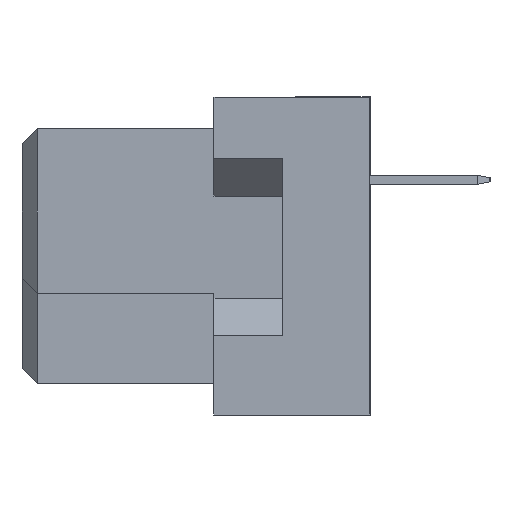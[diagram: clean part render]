
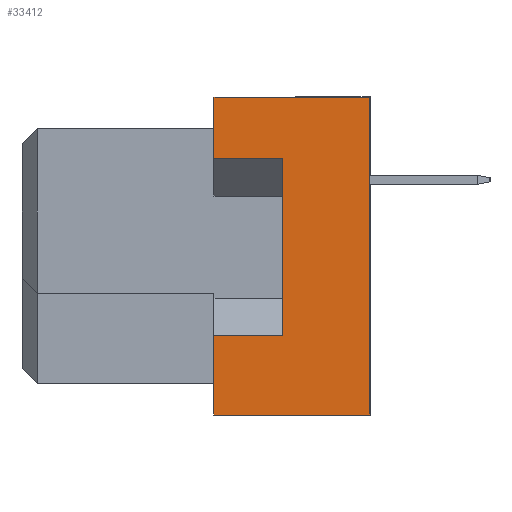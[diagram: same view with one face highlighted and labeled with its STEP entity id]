
A CAD part, left-side view. The second image highlights one B-rep face of the part: STEP entity #33412.
In plain terms, the highlighted planar face has unit normal (-1, 0, 0).
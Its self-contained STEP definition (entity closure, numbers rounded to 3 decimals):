
#523 = PLANE ( 'NONE',  #37031 ) ;
#1334 = ORIENTED_EDGE ( 'NONE', *, *, #15803, .F. ) ;
#2146 = FACE_OUTER_BOUND ( 'NONE', #35616, .T. ) ;
#2546 = CARTESIAN_POINT ( 'NONE',  ( -47.5, -6.4, 3.25 ) ) ;
#2981 = VECTOR ( 'NONE', #35082, 1000. ) ;
#3754 = LINE ( 'NONE', #12073, #26467 ) ;
#3758 = DIRECTION ( 'NONE',  ( 0., 1., 0. ) ) ;
#4935 = CARTESIAN_POINT ( 'NONE',  ( -47.5, -8.7, -2.65 ) ) ;
#5899 = CARTESIAN_POINT ( 'NONE',  ( -47.5, -6.4, -5.3 ) ) ;
#7031 = DIRECTION ( 'NONE',  ( 0., 1., 0. ) ) ;
#7645 = EDGE_CURVE ( 'NONE', #26529, #24232, #8634, .T. ) ;
#8069 = CARTESIAN_POINT ( 'NONE',  ( -47.5, -6.4, -5.3 ) ) ;
#8288 = VERTEX_POINT ( 'NONE', #26738 ) ;
#8634 = LINE ( 'NONE', #8069, #2981 ) ;
#8701 = CARTESIAN_POINT ( 'NONE',  ( -47.5, -8.7, -2.65 ) ) ;
#8948 = CARTESIAN_POINT ( 'NONE',  ( -47.5, -11.6, 5.3 ) ) ;
#9218 = CARTESIAN_POINT ( 'NONE',  ( -47.5, -11.6, 5.3 ) ) ;
#9514 = VERTEX_POINT ( 'NONE', #4935 ) ;
#9532 = VECTOR ( 'NONE', #21009, 1000. ) ;
#10027 = VECTOR ( 'NONE', #21913, 1000. ) ;
#10744 = ORIENTED_EDGE ( 'NONE', *, *, #33076, .T. ) ;
#11091 = CARTESIAN_POINT ( 'NONE',  ( -47.5, -11.6, 5.3 ) ) ;
#12073 = CARTESIAN_POINT ( 'NONE',  ( -47.5, -8.7, 3.25 ) ) ;
#13575 = LINE ( 'NONE', #33482, #10027 ) ;
#13934 = CARTESIAN_POINT ( 'NONE',  ( -47.5, -11.6, 5.3 ) ) ;
#15022 = ORIENTED_EDGE ( 'NONE', *, *, #32211, .T. ) ;
#15739 = CARTESIAN_POINT ( 'NONE',  ( -47.5, -11.6, -5.3 ) ) ;
#15803 = EDGE_CURVE ( 'NONE', #9514, #36334, #23382, .T. ) ;
#15843 = ORIENTED_EDGE ( 'NONE', *, *, #19624, .F. ) ;
#16558 = ORIENTED_EDGE ( 'NONE', *, *, #7645, .F. ) ;
#17599 = DIRECTION ( 'NONE',  ( 0., 0., 1. ) ) ;
#19171 = VECTOR ( 'NONE', #31764, 1000. ) ;
#19624 = EDGE_CURVE ( 'NONE', #36334, #26529, #3754, .T. ) ;
#20251 = LINE ( 'NONE', #9218, #9532 ) ;
#21009 = DIRECTION ( 'NONE',  ( 0., 1., 0. ) ) ;
#21913 = DIRECTION ( 'NONE',  ( 0., 0., 1. ) ) ;
#22422 = CARTESIAN_POINT ( 'NONE',  ( -47.5, -6.4, -2.65 ) ) ;
#22832 = VERTEX_POINT ( 'NONE', #5899 ) ;
#23065 = LINE ( 'NONE', #8948, #19171 ) ;
#23382 = LINE ( 'NONE', #8701, #26138 ) ;
#24232 = VERTEX_POINT ( 'NONE', #32601 ) ;
#24442 = LINE ( 'NONE', #15739, #32780 ) ;
#24655 = ORIENTED_EDGE ( 'NONE', *, *, #29589, .F. ) ;
#26138 = VECTOR ( 'NONE', #17599, 1000. ) ;
#26467 = VECTOR ( 'NONE', #27324, 1000. ) ;
#26529 = VERTEX_POINT ( 'NONE', #2546 ) ;
#26738 = CARTESIAN_POINT ( 'NONE',  ( -47.5, -11.6, -5.3 ) ) ;
#27324 = DIRECTION ( 'NONE',  ( 0., 1., 0. ) ) ;
#27876 = LINE ( 'NONE', #31360, #31622 ) ;
#28430 = VERTEX_POINT ( 'NONE', #22422 ) ;
#28808 = DIRECTION ( 'NONE',  ( -1., 0., 0. ) ) ;
#29589 = EDGE_CURVE ( 'NONE', #22832, #28430, #13575, .T. ) ;
#29601 = EDGE_CURVE ( 'NONE', #9514, #28430, #27876, .T. ) ;
#31360 = CARTESIAN_POINT ( 'NONE',  ( -47.5, -8.7, -2.65 ) ) ;
#31622 = VECTOR ( 'NONE', #7031, 1000. ) ;
#31764 = DIRECTION ( 'NONE',  ( 0., 0., 1. ) ) ;
#31822 = ORIENTED_EDGE ( 'NONE', *, *, #29601, .T. ) ;
#32211 = EDGE_CURVE ( 'NONE', #37098, #24232, #20251, .T. ) ;
#32601 = CARTESIAN_POINT ( 'NONE',  ( -47.5, -6.4, 5.3 ) ) ;
#32780 = VECTOR ( 'NONE', #3758, 1000. ) ;
#33076 = EDGE_CURVE ( 'NONE', #8288, #37098, #23065, .T. ) ;
#33412 = ADVANCED_FACE ( 'NONE', ( #2146 ), #523, .T. ) ;
#33482 = CARTESIAN_POINT ( 'NONE',  ( -47.5, -6.4, -5.3 ) ) ;
#33993 = EDGE_CURVE ( 'NONE', #8288, #22832, #24442, .T. ) ;
#34410 = CARTESIAN_POINT ( 'NONE',  ( -47.5, -8.7, 3.25 ) ) ;
#35082 = DIRECTION ( 'NONE',  ( 0., 0., 1. ) ) ;
#35616 = EDGE_LOOP ( 'NONE', ( #31822, #24655, #36962, #10744, #15022, #16558, #15843, #1334 ) ) ;
#35671 = DIRECTION ( 'NONE',  ( 0., 0., 1. ) ) ;
#36334 = VERTEX_POINT ( 'NONE', #34410 ) ;
#36962 = ORIENTED_EDGE ( 'NONE', *, *, #33993, .F. ) ;
#37031 = AXIS2_PLACEMENT_3D ( 'NONE', #13934, #28808, #35671 ) ;
#37098 = VERTEX_POINT ( 'NONE', #11091 ) ;
